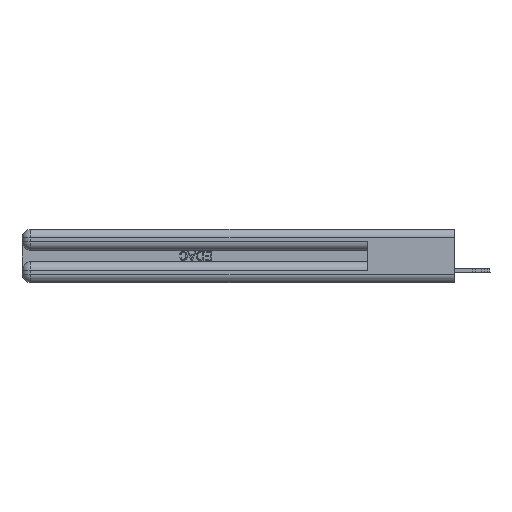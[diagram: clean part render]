
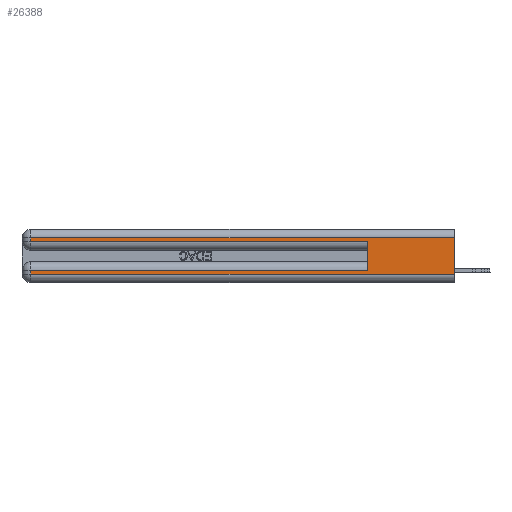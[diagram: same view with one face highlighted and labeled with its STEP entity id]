
A CAD part, left-side view. The second image highlights one B-rep face of the part: STEP entity #26388.
In plain terms, the highlighted planar face has unit normal (-1, 0, 0).
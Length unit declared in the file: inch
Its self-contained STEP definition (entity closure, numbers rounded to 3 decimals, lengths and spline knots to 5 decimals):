
#1056 = VECTOR ( 'NONE', #11556, 39.37008 ) ;
#1429 = CARTESIAN_POINT ( 'NONE',  ( 0., 0., 0.285 ) ) ;
#1678 = VERTEX_POINT ( 'NONE', #40408 ) ;
#1724 = VERTEX_POINT ( 'NONE', #17727 ) ;
#2225 = LINE ( 'NONE', #36715, #31894 ) ;
#2523 = EDGE_CURVE ( 'NONE', #1724, #1678, #38947, .T. ) ;
#2875 = ORIENTED_EDGE ( 'NONE', *, *, #12447, .T. ) ;
#2911 = VERTEX_POINT ( 'NONE', #4915 ) ;
#3827 = DIRECTION ( 'NONE',  ( 0., 0., -1. ) ) ;
#3836 = VECTOR ( 'NONE', #17661, 39.37008 ) ;
#4123 = VERTEX_POINT ( 'NONE', #31629 ) ;
#4725 = ORIENTED_EDGE ( 'NONE', *, *, #42294, .T. ) ;
#4915 = CARTESIAN_POINT ( 'NONE',  ( 0., 0., 0.06 ) ) ;
#5271 = LINE ( 'NONE', #38736, #38987 ) ;
#5680 = EDGE_CURVE ( 'NONE', #15053, #2911, #7151, .T. ) ;
#7151 = LINE ( 'NONE', #22066, #14910 ) ;
#7232 = CARTESIAN_POINT ( 'NONE',  ( 0., 0., 0.37 ) ) ;
#8666 = ORIENTED_EDGE ( 'NONE', *, *, #2523, .T. ) ;
#9537 = EDGE_CURVE ( 'NONE', #1724, #28033, #13491, .T. ) ;
#10787 = VECTOR ( 'NONE', #30616, 39.37008 ) ;
#11556 = DIRECTION ( 'NONE',  ( 0., 1., 0. ) ) ;
#11975 = CARTESIAN_POINT ( 'NONE',  ( 0., 0.6, 0.285 ) ) ;
#12447 = EDGE_CURVE ( 'NONE', #36691, #39088, #2225, .T. ) ;
#12880 = EDGE_CURVE ( 'NONE', #39088, #28033, #30808, .T. ) ;
#13491 = LINE ( 'NONE', #40384, #31946 ) ;
#14037 = CARTESIAN_POINT ( 'NONE',  ( 0., 0., 0.085 ) ) ;
#14910 = VECTOR ( 'NONE', #35113, 39.37008 ) ;
#15053 = VERTEX_POINT ( 'NONE', #20705 ) ;
#16175 = LINE ( 'NONE', #36786, #3836 ) ;
#17661 = DIRECTION ( 'NONE',  ( 0., -1., 0. ) ) ;
#17727 = CARTESIAN_POINT ( 'NONE',  ( 0., 0.6, 0.085 ) ) ;
#17991 = ORIENTED_EDGE ( 'NONE', *, *, #5680, .F. ) ;
#17996 = CARTESIAN_POINT ( 'NONE',  ( 0., 0., 0.31 ) ) ;
#18267 = ORIENTED_EDGE ( 'NONE', *, *, #9537, .F. ) ;
#18745 = FACE_OUTER_BOUND ( 'NONE', #40638, .T. ) ;
#20404 = PLANE ( 'NONE',  #26624 ) ;
#20705 = CARTESIAN_POINT ( 'NONE',  ( 0., 0., 0.31 ) ) ;
#20808 = DIRECTION ( 'NONE',  ( 0., 0., 1. ) ) ;
#22066 = CARTESIAN_POINT ( 'NONE',  ( 0., 0., 0.37 ) ) ;
#23564 = LINE ( 'NONE', #17996, #1056 ) ;
#26388 = ADVANCED_FACE ( 'NONE', ( #18745 ), #20404, .F. ) ;
#26465 = ORIENTED_EDGE ( 'NONE', *, *, #30964, .T. ) ;
#26624 = AXIS2_PLACEMENT_3D ( 'NONE', #7232, #27156, #26707 ) ;
#26707 = DIRECTION ( 'NONE',  ( 0., 0., -1. ) ) ;
#27156 = DIRECTION ( 'NONE',  ( 1., 0., 0. ) ) ;
#28033 = VERTEX_POINT ( 'NONE', #11975 ) ;
#28921 = DIRECTION ( 'NONE',  ( 0., 0., -1. ) ) ;
#30616 = DIRECTION ( 'NONE',  ( 0., 1., 0. ) ) ;
#30808 = LINE ( 'NONE', #1429, #35916 ) ;
#30964 = EDGE_CURVE ( 'NONE', #15053, #36691, #23564, .T. ) ;
#31629 = CARTESIAN_POINT ( 'NONE',  ( 0., 2.94, 0.06 ) ) ;
#31894 = VECTOR ( 'NONE', #3827, 39.37008 ) ;
#31946 = VECTOR ( 'NONE', #20808, 39.37008 ) ;
#35113 = DIRECTION ( 'NONE',  ( 0., 0., -1. ) ) ;
#35916 = VECTOR ( 'NONE', #37298, 39.37008 ) ;
#36691 = VERTEX_POINT ( 'NONE', #36941 ) ;
#36715 = CARTESIAN_POINT ( 'NONE',  ( 0., 2.94, 0.37 ) ) ;
#36786 = CARTESIAN_POINT ( 'NONE',  ( 0., 0., 0.06 ) ) ;
#36941 = CARTESIAN_POINT ( 'NONE',  ( 0., 2.94, 0.31 ) ) ;
#37214 = ORIENTED_EDGE ( 'NONE', *, *, #38942, .T. ) ;
#37298 = DIRECTION ( 'NONE',  ( 0., -1., 0. ) ) ;
#38736 = CARTESIAN_POINT ( 'NONE',  ( 0., 2.94, 0.37 ) ) ;
#38942 = EDGE_CURVE ( 'NONE', #1678, #4123, #5271, .T. ) ;
#38947 = LINE ( 'NONE', #14037, #10787 ) ;
#38987 = VECTOR ( 'NONE', #28921, 39.37008 ) ;
#39088 = VERTEX_POINT ( 'NONE', #39785 ) ;
#39401 = ORIENTED_EDGE ( 'NONE', *, *, #12880, .T. ) ;
#39785 = CARTESIAN_POINT ( 'NONE',  ( 0., 2.94, 0.285 ) ) ;
#40384 = CARTESIAN_POINT ( 'NONE',  ( 0., 0.6, 0.145 ) ) ;
#40408 = CARTESIAN_POINT ( 'NONE',  ( 0., 2.94, 0.085 ) ) ;
#40638 = EDGE_LOOP ( 'NONE', ( #17991, #26465, #2875, #39401, #18267, #8666, #37214, #4725 ) ) ;
#42294 = EDGE_CURVE ( 'NONE', #4123, #2911, #16175, .T. ) ;
